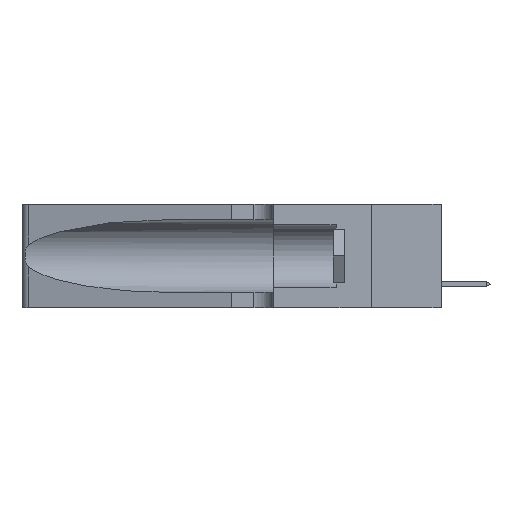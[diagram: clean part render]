
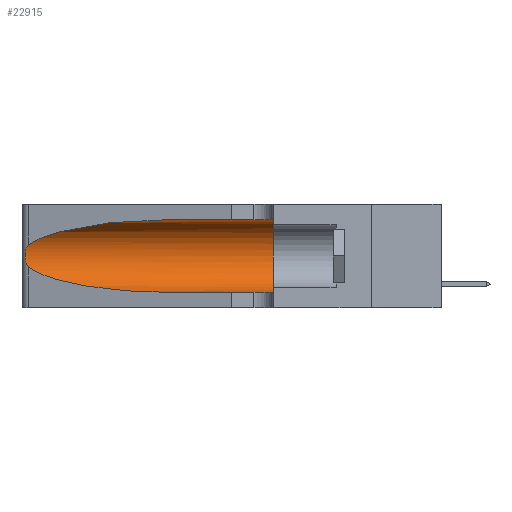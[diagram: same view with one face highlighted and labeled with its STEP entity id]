
A CAD part, left-side view. The second image highlights one B-rep face of the part: STEP entity #22915.
In plain terms, the highlighted cylindrical face has radius 3.308 mm (diameter 6.617 mm), a partial arc.
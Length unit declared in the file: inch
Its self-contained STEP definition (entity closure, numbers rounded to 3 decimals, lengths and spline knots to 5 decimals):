
#1835 = DIRECTION ( 'NONE',  ( 0., -1., 0. ) ) ;
#2473 = CYLINDRICAL_SURFACE ( 'NONE', #20918, 0.13025 ) ;
#2935 = CARTESIAN_POINT ( 'NONE',  ( 0.25639, 1.23186, 0.15144 ) ) ;
#3438 = VERTEX_POINT ( 'NONE', #47138 ) ;
#3562 = VERTEX_POINT ( 'NONE', #20577 ) ;
#3774 = ORIENTED_EDGE ( 'NONE', *, *, #47833, .F. ) ;
#5755 = DIRECTION ( 'NONE',  ( 0., 0., -1. ) ) ;
#6318 = CARTESIAN_POINT ( 'NONE',  ( 0.1305, 0.72297, 0.31525 ) ) ;
#6333 = DIRECTION ( 'NONE',  ( 0., 1., 0. ) ) ;
#6657 = CARTESIAN_POINT ( 'NONE',  ( 0.26075, 1.23896, 0.19203 ) ) ;
#7788 = ORIENTED_EDGE ( 'NONE', *, *, #44564, .T. ) ;
#8188 = CARTESIAN_POINT ( 'NONE',  ( 0.2373, 1.15595, 0.08982 ) ) ;
#8496 = LINE ( 'NONE', #37039, #47421 ) ;
#9337 = CARTESIAN_POINT ( 'NONE',  ( 0.1305, 0.35, 0.31525 ) ) ;
#9469 = FACE_OUTER_BOUND ( 'NONE', #12753, .T. ) ;
#10038 = CARTESIAN_POINT ( 'NONE',  ( 0.1305, 0.72297, 0.31525 ) ) ;
#10210 = CARTESIAN_POINT ( 'NONE',  ( 0.25487, 1.22718, 0.22369 ) ) ;
#10896 = CARTESIAN_POINT ( 'NONE',  ( 0.25487, 1.22718, 0.22369 ) ) ;
#11044 = CARTESIAN_POINT ( 'NONE',  ( 0.26018, 1.23835, 0.19895 ) ) ;
#11526 = VERTEX_POINT ( 'NONE', #24613 ) ;
#12753 = EDGE_LOOP ( 'NONE', ( #33662, #7788, #31507, #29828, #3774, #22187 ) ) ;
#14338 = EDGE_CURVE ( 'NONE', #3438, #47532, #8496, .T. ) ;
#14448 = B_SPLINE_CURVE_WITH_KNOTS ( 'NONE', 3,
 ( #10896, #29796, #36923, #33604, #37403, #11044, #6657, #14788, #18574, #22366, #40739, #2935, #32948, #37079 ),
 .UNSPECIFIED., .F., .F.,
 ( 4, 2, 2, 2, 2, 2, 4 ),
 ( 0., 0.00027, 0.00053, 0.00107, 0.0016, 0.00187, 0.00214 ),
 .UNSPECIFIED. ) ;
#14788 = CARTESIAN_POINT ( 'NONE',  ( 0.26075, 1.23896, 0.178 ) ) ;
#17756 = CARTESIAN_POINT ( 'NONE',  ( 0.18966, 0.96281, 0.31525 ) ) ;
#18574 = CARTESIAN_POINT ( 'NONE',  ( 0.26017, 1.23833, 0.17102 ) ) ;
#19571 = EDGE_CURVE ( 'NONE', #3562, #3438, #45056, .T. ) ;
#20577 = CARTESIAN_POINT ( 'NONE',  ( 0.25487, 1.22718, 0.14631 ) ) ;
#20918 = AXIS2_PLACEMENT_3D ( 'NONE', #32515, #1835, #5755 ) ;
#22187 = ORIENTED_EDGE ( 'NONE', *, *, #37085, .F. ) ;
#22366 = CARTESIAN_POINT ( 'NONE',  ( 0.25856, 1.23593, 0.16098 ) ) ;
#22915 = ADVANCED_FACE ( 'NONE', ( #9469 ), #2473, .F. ) ;
#24613 = CARTESIAN_POINT ( 'NONE',  ( 0.25487, 1.22718, 0.22369 ) ) ;
#26249 = VERTEX_POINT ( 'NONE', #10038 ) ;
#26585 = CARTESIAN_POINT ( 'NONE',  ( 0.1305, 1.61858, 0.31525 ) ) ;
#26620 = CARTESIAN_POINT ( 'NONE',  ( 0.1305, 0.35, 0.05475 ) ) ;
#28642 = CARTESIAN_POINT ( 'NONE',  ( 0.2373, 1.15595, 0.28018 ) ) ;
#29712 = VERTEX_POINT ( 'NONE', #9337 ) ;
#29796 = CARTESIAN_POINT ( 'NONE',  ( 0.25555, 1.22994, 0.2215 ) ) ;
#29828 = ORIENTED_EDGE ( 'NONE', *, *, #14338, .T. ) ;
#31288 = VECTOR ( 'NONE', #45599, 39.37008 ) ;
#31507 = ORIENTED_EDGE ( 'NONE', *, *, #19571, .T. ) ;
#31875 = CIRCLE ( 'NONE', #41328, 0.13025 ) ;
#31948 = CARTESIAN_POINT ( 'NONE',  ( 0.1305, 0.35, 0.185 ) ) ;
#32197 = EDGE_CURVE ( 'NONE', #26249, #11526, #40795, .T. ) ;
#32515 = CARTESIAN_POINT ( 'NONE',  ( 0.1305, 1.61858, 0.185 ) ) ;
#32948 = CARTESIAN_POINT ( 'NONE',  ( 0.25555, 1.22993, 0.14849 ) ) ;
#33604 = CARTESIAN_POINT ( 'NONE',  ( 0.25787, 1.23484, 0.2124 ) ) ;
#33662 = ORIENTED_EDGE ( 'NONE', *, *, #32197, .T. ) ;
#34488 = CARTESIAN_POINT ( 'NONE',  ( 0.1305, 0.72297, 0.05475 ) ) ;
#36923 = CARTESIAN_POINT ( 'NONE',  ( 0.25639, 1.23184, 0.21858 ) ) ;
#37039 = CARTESIAN_POINT ( 'NONE',  ( 0.1305, 1.61858, 0.05475 ) ) ;
#37079 = CARTESIAN_POINT ( 'NONE',  ( 0.25487, 1.22718, 0.14631 ) ) ;
#37085 = EDGE_CURVE ( 'NONE', #26249, #29712, #38336, .T. ) ;
#37403 = CARTESIAN_POINT ( 'NONE',  ( 0.25854, 1.2359, 0.20912 ) ) ;
#38336 = LINE ( 'NONE', #26585, #31288 ) ;
#39546 = DIRECTION ( 'NONE',  ( 0., 0., 1. ) ) ;
#40739 = CARTESIAN_POINT ( 'NONE',  ( 0.25789, 1.23486, 0.15765 ) ) ;
#40795 =( BOUNDED_CURVE ( )  B_SPLINE_CURVE ( 3, ( #6318, #17756, #28642, #10210 ),
 .UNSPECIFIED., .F., .T. ) 
 B_SPLINE_CURVE_WITH_KNOTS ( ( 4, 4 ),
 ( 1.5708, 2.84003 ),
 .UNSPECIFIED. ) 
 CURVE ( )  GEOMETRIC_REPRESENTATION_ITEM ( )  RATIONAL_B_SPLINE_CURVE ( ( 1., 0.87, 0.87, 1. ) ) 
 REPRESENTATION_ITEM ( '' )  );
#41029 = DIRECTION ( 'NONE',  ( 0., -1., 0. ) ) ;
#41167 = CARTESIAN_POINT ( 'NONE',  ( 0.25487, 1.22718, 0.14631 ) ) ;
#41328 = AXIS2_PLACEMENT_3D ( 'NONE', #31948, #6333, #39546 ) ;
#44564 = EDGE_CURVE ( 'NONE', #11526, #3562, #14448, .T. ) ;
#45056 =( BOUNDED_CURVE ( )  B_SPLINE_CURVE ( 3, ( #41167, #8188, #45765, #34488 ),
 .UNSPECIFIED., .F., .T. ) 
 B_SPLINE_CURVE_WITH_KNOTS ( ( 4, 4 ),
 ( 3.44316, 4.71239 ),
 .UNSPECIFIED. ) 
 CURVE ( )  GEOMETRIC_REPRESENTATION_ITEM ( )  RATIONAL_B_SPLINE_CURVE ( ( 1., 0.87, 0.87, 1. ) ) 
 REPRESENTATION_ITEM ( '' )  );
#45599 = DIRECTION ( 'NONE',  ( 0., -1., 0. ) ) ;
#45765 = CARTESIAN_POINT ( 'NONE',  ( 0.18966, 0.96281, 0.05475 ) ) ;
#47138 = CARTESIAN_POINT ( 'NONE',  ( 0.1305, 0.72297, 0.05475 ) ) ;
#47421 = VECTOR ( 'NONE', #41029, 39.37008 ) ;
#47532 = VERTEX_POINT ( 'NONE', #26620 ) ;
#47833 = EDGE_CURVE ( 'NONE', #29712, #47532, #31875, .T. ) ;
